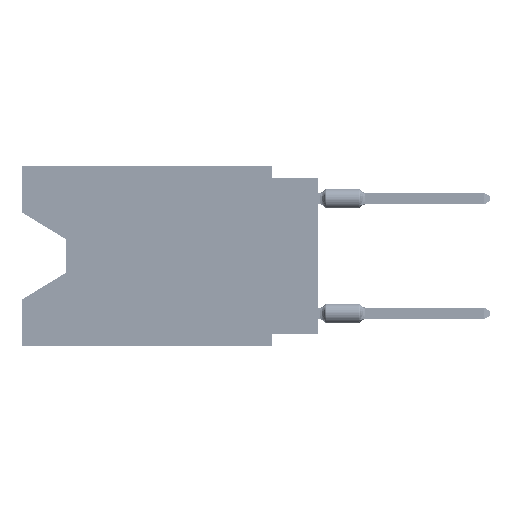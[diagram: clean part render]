
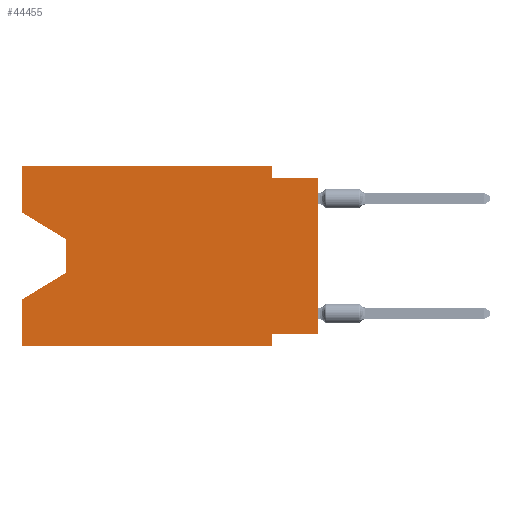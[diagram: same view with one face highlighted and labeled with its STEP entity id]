
A CAD part, left-side view. The second image highlights one B-rep face of the part: STEP entity #44455.
In plain terms, the highlighted planar face has unit normal (-1, 0, 0).
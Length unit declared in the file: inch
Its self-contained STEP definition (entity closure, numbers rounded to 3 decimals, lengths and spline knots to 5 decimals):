
#28 = LINE ( 'NONE', #11583, #18333 ) ;
#1090 = EDGE_CURVE ( 'NONE', #69793, #39011, #46244, .T. ) ;
#2771 = EDGE_CURVE ( 'NONE', #41124, #68174, #24556, .T. ) ;
#3394 = CARTESIAN_POINT ( 'NONE',  ( 0., 0.1, -0.39 ) ) ;
#3953 = VECTOR ( 'NONE', #52395, 39.37008 ) ;
#4007 = ORIENTED_EDGE ( 'NONE', *, *, #50247, .F. ) ;
#4091 = EDGE_CURVE ( 'NONE', #57006, #40594, #11877, .T. ) ;
#4651 = CARTESIAN_POINT ( 'NONE',  ( 0., 0.645, 0. ) ) ;
#5351 = CARTESIAN_POINT ( 'NONE',  ( 0., 0., -0.025 ) ) ;
#6279 = VERTEX_POINT ( 'NONE', #65770 ) ;
#7027 = AXIS2_PLACEMENT_3D ( 'NONE', #22972, #22187, #28731 ) ;
#8779 = CARTESIAN_POINT ( 'NONE',  ( 0., 0., -0.365 ) ) ;
#11172 = DIRECTION ( 'NONE',  ( 0., 0., 1. ) ) ;
#11583 = CARTESIAN_POINT ( 'NONE',  ( 0., 0., 0. ) ) ;
#11877 = LINE ( 'NONE', #5351, #14090 ) ;
#12920 = VECTOR ( 'NONE', #11172, 39.37008 ) ;
#13408 = DIRECTION ( 'NONE',  ( 0., 1., 0. ) ) ;
#13623 = ORIENTED_EDGE ( 'NONE', *, *, #62274, .T. ) ;
#14090 = VECTOR ( 'NONE', #23794, 39.37008 ) ;
#14166 = VERTEX_POINT ( 'NONE', #18651 ) ;
#14688 = VERTEX_POINT ( 'NONE', #54706 ) ;
#15376 = VERTEX_POINT ( 'NONE', #64587 ) ;
#18332 = VERTEX_POINT ( 'NONE', #67262 ) ;
#18333 = VECTOR ( 'NONE', #23497, 39.37008 ) ;
#18651 = CARTESIAN_POINT ( 'NONE',  ( 0., 0., -0.365 ) ) ;
#18978 = VECTOR ( 'NONE', #66808, 39.37008 ) ;
#19556 = CARTESIAN_POINT ( 'NONE',  ( 0., 0.645, 0. ) ) ;
#19865 = LINE ( 'NONE', #43311, #18978 ) ;
#22126 = EDGE_CURVE ( 'NONE', #14166, #15376, #36875, .T. ) ;
#22187 = DIRECTION ( 'NONE',  ( 1., 0., 0. ) ) ;
#22972 = CARTESIAN_POINT ( 'NONE',  ( 0., 0.645, 0. ) ) ;
#22981 = VECTOR ( 'NONE', #43383, 39.37008 ) ;
#23038 = VECTOR ( 'NONE', #67258, 39.37008 ) ;
#23373 = EDGE_CURVE ( 'NONE', #18332, #14688, #55718, .T. ) ;
#23497 = DIRECTION ( 'NONE',  ( 0., 0., 1. ) ) ;
#23794 = DIRECTION ( 'NONE',  ( 0., -1., 0. ) ) ;
#24556 = LINE ( 'NONE', #19556, #22981 ) ;
#28683 = VERTEX_POINT ( 'NONE', #3394 ) ;
#28731 = DIRECTION ( 'NONE',  ( 0., 0., -1. ) ) ;
#28926 = CARTESIAN_POINT ( 'NONE',  ( 0., 0.645, 0. ) ) ;
#29563 = ORIENTED_EDGE ( 'NONE', *, *, #30566, .T. ) ;
#30566 = EDGE_CURVE ( 'NONE', #14688, #6279, #49367, .T. ) ;
#33492 = LINE ( 'NONE', #4651, #12920 ) ;
#33665 = VECTOR ( 'NONE', #51775, 39.37008 ) ;
#36169 = ORIENTED_EDGE ( 'NONE', *, *, #38885, .T. ) ;
#36875 = LINE ( 'NONE', #8779, #55202 ) ;
#37032 = LINE ( 'NONE', #54729, #48051 ) ;
#37856 = EDGE_LOOP ( 'NONE', ( #52368, #29563, #38952, #59959, #36169, #54124, #65052, #13623, #44509, #4007, #50068, #70002 ) ) ;
#38885 = EDGE_CURVE ( 'NONE', #69793, #28683, #73071, .T. ) ;
#38952 = ORIENTED_EDGE ( 'NONE', *, *, #53838, .T. ) ;
#39011 = VERTEX_POINT ( 'NONE', #52543 ) ;
#40594 = VERTEX_POINT ( 'NONE', #62149 ) ;
#41124 = VERTEX_POINT ( 'NONE', #68586 ) ;
#42488 = DIRECTION ( 'NONE',  ( 0., 0., -1. ) ) ;
#43311 = CARTESIAN_POINT ( 'NONE',  ( 0., 0.55, -0.232 ) ) ;
#43383 = DIRECTION ( 'NONE',  ( 0., -1., 0. ) ) ;
#44455 = ADVANCED_FACE ( 'NONE', ( #63390 ), #69901, .F. ) ;
#44509 = ORIENTED_EDGE ( 'NONE', *, *, #4091, .F. ) ;
#46244 = LINE ( 'NONE', #28926, #3953 ) ;
#47928 = CARTESIAN_POINT ( 'NONE',  ( 0., 0.645, -0.39 ) ) ;
#48051 = VECTOR ( 'NONE', #67796, 39.37008 ) ;
#48488 = VECTOR ( 'NONE', #42488, 39.37008 ) ;
#49367 = LINE ( 'NONE', #72861, #48488 ) ;
#50068 = ORIENTED_EDGE ( 'NONE', *, *, #2771, .F. ) ;
#50247 = EDGE_CURVE ( 'NONE', #68174, #57006, #37032, .T. ) ;
#51775 = DIRECTION ( 'NONE',  ( 0., -1., 0. ) ) ;
#52368 = ORIENTED_EDGE ( 'NONE', *, *, #23373, .T. ) ;
#52395 = DIRECTION ( 'NONE',  ( 0., 0., 1. ) ) ;
#52543 = CARTESIAN_POINT ( 'NONE',  ( 0., 0.645, -0.28975 ) ) ;
#53607 = CARTESIAN_POINT ( 'NONE',  ( 0., 0.1, -0.025 ) ) ;
#53838 = EDGE_CURVE ( 'NONE', #6279, #39011, #19865, .T. ) ;
#54124 = ORIENTED_EDGE ( 'NONE', *, *, #59145, .F. ) ;
#54549 = CARTESIAN_POINT ( 'NONE',  ( 0., 0.1, -0.39 ) ) ;
#54706 = CARTESIAN_POINT ( 'NONE',  ( 0., 0.55, -0.158 ) ) ;
#54729 = CARTESIAN_POINT ( 'NONE',  ( 0., 0.1, 0. ) ) ;
#54947 = EDGE_CURVE ( 'NONE', #18332, #41124, #33492, .T. ) ;
#55202 = VECTOR ( 'NONE', #13408, 39.37008 ) ;
#55718 = LINE ( 'NONE', #67662, #62738 ) ;
#57006 = VERTEX_POINT ( 'NONE', #53607 ) ;
#57168 = CARTESIAN_POINT ( 'NONE',  ( 0., 0.645, -0.39 ) ) ;
#59145 = EDGE_CURVE ( 'NONE', #15376, #28683, #72625, .T. ) ;
#59959 = ORIENTED_EDGE ( 'NONE', *, *, #1090, .F. ) ;
#62149 = CARTESIAN_POINT ( 'NONE',  ( 0., 0., -0.025 ) ) ;
#62274 = EDGE_CURVE ( 'NONE', #14166, #40594, #28, .T. ) ;
#62738 = VECTOR ( 'NONE', #72662, 39.37008 ) ;
#63390 = FACE_OUTER_BOUND ( 'NONE', #37856, .T. ) ;
#64587 = CARTESIAN_POINT ( 'NONE',  ( 0., 0.1, -0.365 ) ) ;
#65052 = ORIENTED_EDGE ( 'NONE', *, *, #22126, .F. ) ;
#65770 = CARTESIAN_POINT ( 'NONE',  ( 0., 0.55, -0.232 ) ) ;
#66782 = CARTESIAN_POINT ( 'NONE',  ( 0., 0.1, 0. ) ) ;
#66808 = DIRECTION ( 'NONE',  ( 0., 0.855, -0.519 ) ) ;
#67258 = DIRECTION ( 'NONE',  ( 0., 0., -1. ) ) ;
#67262 = CARTESIAN_POINT ( 'NONE',  ( 0., 0.645, -0.10025 ) ) ;
#67662 = CARTESIAN_POINT ( 'NONE',  ( 0., 0.645, -0.10025 ) ) ;
#67796 = DIRECTION ( 'NONE',  ( 0., 0., -1. ) ) ;
#68174 = VERTEX_POINT ( 'NONE', #66782 ) ;
#68586 = CARTESIAN_POINT ( 'NONE',  ( 0., 0.645, 0. ) ) ;
#69793 = VERTEX_POINT ( 'NONE', #47928 ) ;
#69901 = PLANE ( 'NONE',  #7027 ) ;
#70002 = ORIENTED_EDGE ( 'NONE', *, *, #54947, .F. ) ;
#72625 = LINE ( 'NONE', #54549, #23038 ) ;
#72662 = DIRECTION ( 'NONE',  ( 0., -0.855, -0.519 ) ) ;
#72861 = CARTESIAN_POINT ( 'NONE',  ( 0., 0.55, -0.158 ) ) ;
#73071 = LINE ( 'NONE', #57168, #33665 ) ;
